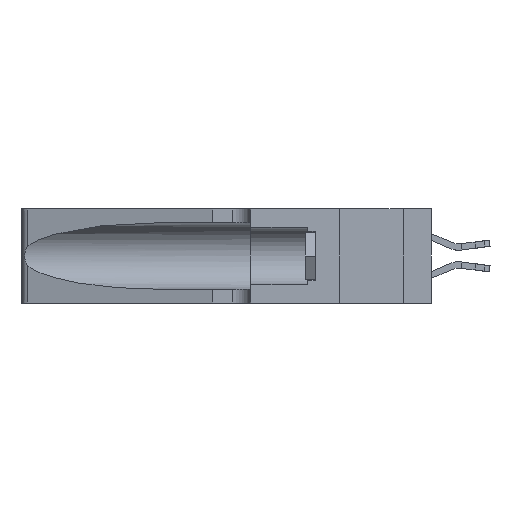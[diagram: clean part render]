
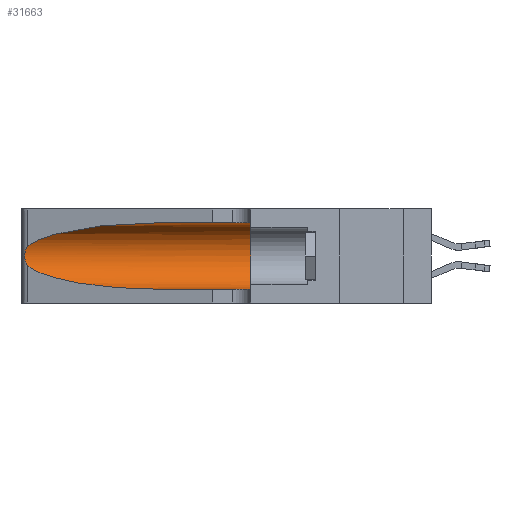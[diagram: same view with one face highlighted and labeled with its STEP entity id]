
A CAD part, left-side view. The second image highlights one B-rep face of the part: STEP entity #31663.
In plain terms, the highlighted cylindrical face has radius 3.308 mm (diameter 6.617 mm), a partial arc.
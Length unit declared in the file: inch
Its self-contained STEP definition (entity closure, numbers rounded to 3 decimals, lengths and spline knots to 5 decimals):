
#48 = AXIS2_PLACEMENT_3D ( 'NONE', #29985, #5569, #8270 ) ;
#998 = DIRECTION ( 'NONE',  ( 0., 0., 1. ) ) ;
#1573 = DIRECTION ( 'NONE',  ( 0., -1., 0. ) ) ;
#1685 = CARTESIAN_POINT ( 'NONE',  ( 0.18966, 0.96281, 0.31525 ) ) ;
#1774 = CARTESIAN_POINT ( 'NONE',  ( 0.25856, 1.23593, 0.16098 ) ) ;
#2939 = CARTESIAN_POINT ( 'NONE',  ( 0.25487, 1.22718, 0.22369 ) ) ;
#3150 = VERTEX_POINT ( 'NONE', #20504 ) ;
#4225 = CARTESIAN_POINT ( 'NONE',  ( 0.25789, 1.23486, 0.15765 ) ) ;
#4464 = EDGE_CURVE ( 'NONE', #17666, #22763, #25369, .T. ) ;
#5317 = ORIENTED_EDGE ( 'NONE', *, *, #5545, .T. ) ;
#5545 = EDGE_CURVE ( 'NONE', #11251, #17666, #10088, .T. ) ;
#5569 = DIRECTION ( 'NONE',  ( 0., -1., 0. ) ) ;
#6688 = CARTESIAN_POINT ( 'NONE',  ( 0.1305, 1.61858, 0.31525 ) ) ;
#7554 = CARTESIAN_POINT ( 'NONE',  ( 0.1305, 0.72297, 0.05475 ) ) ;
#8163 = DIRECTION ( 'NONE',  ( 0., 1., 0. ) ) ;
#8270 = DIRECTION ( 'NONE',  ( 0., 0., -1. ) ) ;
#8498 = CARTESIAN_POINT ( 'NONE',  ( 0.1305, 0.72297, 0.05475 ) ) ;
#8927 = VECTOR ( 'NONE', #1573, 39.37008 ) ;
#8980 = EDGE_CURVE ( 'NONE', #22763, #3150, #30144, .T. ) ;
#10037 = LINE ( 'NONE', #6688, #8927 ) ;
#10088 = B_SPLINE_CURVE_WITH_KNOTS ( 'NONE', 3,
 ( #2939, #12464, #25858, #18370, #28415, #28521, #13785, #31165, #30872, #1774, #4225, #12125, #22080, #19556 ),
 .UNSPECIFIED., .F., .F.,
 ( 4, 2, 2, 2, 2, 2, 4 ),
 ( 0., 0.00027, 0.00053, 0.00107, 0.0016, 0.00187, 0.00214 ),
 .UNSPECIFIED. ) ;
#10791 = CARTESIAN_POINT ( 'NONE',  ( 0.25487, 1.22718, 0.14631 ) ) ;
#10794 = ORIENTED_EDGE ( 'NONE', *, *, #23652, .F. ) ;
#11251 = VERTEX_POINT ( 'NONE', #30845 ) ;
#11323 = CARTESIAN_POINT ( 'NONE',  ( 0.25487, 1.22718, 0.22369 ) ) ;
#12125 = CARTESIAN_POINT ( 'NONE',  ( 0.25639, 1.23186, 0.15144 ) ) ;
#12464 = CARTESIAN_POINT ( 'NONE',  ( 0.25555, 1.22994, 0.2215 ) ) ;
#13785 = CARTESIAN_POINT ( 'NONE',  ( 0.26075, 1.23896, 0.19203 ) ) ;
#14408 = EDGE_CURVE ( 'NONE', #21071, #11251, #31457, .T. ) ;
#14700 = ORIENTED_EDGE ( 'NONE', *, *, #8980, .T. ) ;
#14767 = VERTEX_POINT ( 'NONE', #22920 ) ;
#15889 = FACE_OUTER_BOUND ( 'NONE', #30574, .T. ) ;
#17666 = VERTEX_POINT ( 'NONE', #10791 ) ;
#18313 = ORIENTED_EDGE ( 'NONE', *, *, #24931, .F. ) ;
#18362 = CARTESIAN_POINT ( 'NONE',  ( 0.18966, 0.96281, 0.05475 ) ) ;
#18370 = CARTESIAN_POINT ( 'NONE',  ( 0.25787, 1.23484, 0.2124 ) ) ;
#18481 = CARTESIAN_POINT ( 'NONE',  ( 0.25487, 1.22718, 0.14631 ) ) ;
#19556 = CARTESIAN_POINT ( 'NONE',  ( 0.25487, 1.22718, 0.14631 ) ) ;
#20504 = CARTESIAN_POINT ( 'NONE',  ( 0.1305, 0.35, 0.05475 ) ) ;
#20601 = CARTESIAN_POINT ( 'NONE',  ( 0.1305, 0.35, 0.185 ) ) ;
#21071 = VERTEX_POINT ( 'NONE', #31430 ) ;
#22080 = CARTESIAN_POINT ( 'NONE',  ( 0.25555, 1.22993, 0.14849 ) ) ;
#22396 = CIRCLE ( 'NONE', #27199, 0.13025 ) ;
#22763 = VERTEX_POINT ( 'NONE', #7554 ) ;
#22920 = CARTESIAN_POINT ( 'NONE',  ( 0.1305, 0.35, 0.31525 ) ) ;
#23398 = CARTESIAN_POINT ( 'NONE',  ( 0.2373, 1.15595, 0.28018 ) ) ;
#23652 = EDGE_CURVE ( 'NONE', #14767, #3150, #22396, .T. ) ;
#24018 = CARTESIAN_POINT ( 'NONE',  ( 0.1305, 1.61858, 0.05475 ) ) ;
#24931 = EDGE_CURVE ( 'NONE', #21071, #14767, #10037, .T. ) ;
#25369 =( BOUNDED_CURVE ( )  B_SPLINE_CURVE ( 3, ( #18481, #28407, #18362, #8498 ),
 .UNSPECIFIED., .F., .F. ) 
 B_SPLINE_CURVE_WITH_KNOTS ( ( 4, 4 ),
 ( 3.44316, 4.71239 ),
 .UNSPECIFIED. ) 
 CURVE ( )  GEOMETRIC_REPRESENTATION_ITEM ( )  RATIONAL_B_SPLINE_CURVE ( ( 1., 0.87, 0.87, 1. ) ) 
 REPRESENTATION_ITEM ( '' )  );
#25858 = CARTESIAN_POINT ( 'NONE',  ( 0.25639, 1.23184, 0.21858 ) ) ;
#26753 = VECTOR ( 'NONE', #28925, 39.37008 ) ;
#27199 = AXIS2_PLACEMENT_3D ( 'NONE', #20601, #8163, #998 ) ;
#27348 = ORIENTED_EDGE ( 'NONE', *, *, #4464, .T. ) ;
#27723 = CYLINDRICAL_SURFACE ( 'NONE', #48, 0.13025 ) ;
#28407 = CARTESIAN_POINT ( 'NONE',  ( 0.2373, 1.15595, 0.08982 ) ) ;
#28415 = CARTESIAN_POINT ( 'NONE',  ( 0.25854, 1.2359, 0.20912 ) ) ;
#28521 = CARTESIAN_POINT ( 'NONE',  ( 0.26018, 1.23835, 0.19895 ) ) ;
#28536 = CARTESIAN_POINT ( 'NONE',  ( 0.1305, 0.72297, 0.31525 ) ) ;
#28925 = DIRECTION ( 'NONE',  ( 0., -1., 0. ) ) ;
#29985 = CARTESIAN_POINT ( 'NONE',  ( 0.1305, 1.61858, 0.185 ) ) ;
#30144 = LINE ( 'NONE', #24018, #26753 ) ;
#30366 = ORIENTED_EDGE ( 'NONE', *, *, #14408, .T. ) ;
#30574 = EDGE_LOOP ( 'NONE', ( #30366, #5317, #27348, #14700, #10794, #18313 ) ) ;
#30845 = CARTESIAN_POINT ( 'NONE',  ( 0.25487, 1.22718, 0.22369 ) ) ;
#30872 = CARTESIAN_POINT ( 'NONE',  ( 0.26017, 1.23833, 0.17102 ) ) ;
#31165 = CARTESIAN_POINT ( 'NONE',  ( 0.26075, 1.23896, 0.178 ) ) ;
#31430 = CARTESIAN_POINT ( 'NONE',  ( 0.1305, 0.72297, 0.31525 ) ) ;
#31457 =( BOUNDED_CURVE ( )  B_SPLINE_CURVE ( 3, ( #28536, #1685, #23398, #11323 ),
 .UNSPECIFIED., .F., .T. ) 
 B_SPLINE_CURVE_WITH_KNOTS ( ( 4, 4 ),
 ( 1.5708, 2.84003 ),
 .UNSPECIFIED. ) 
 CURVE ( )  GEOMETRIC_REPRESENTATION_ITEM ( )  RATIONAL_B_SPLINE_CURVE ( ( 1., 0.87, 0.87, 1. ) ) 
 REPRESENTATION_ITEM ( '' )  );
#31663 = ADVANCED_FACE ( 'NONE', ( #15889 ), #27723, .F. ) ;
